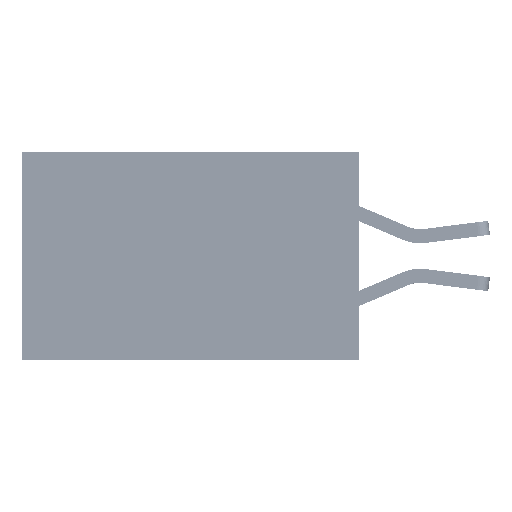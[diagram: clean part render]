
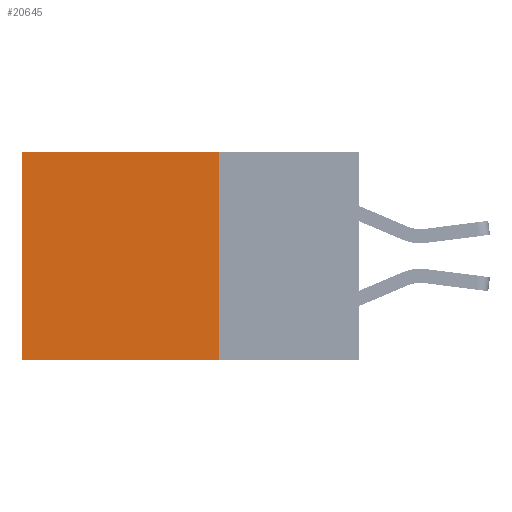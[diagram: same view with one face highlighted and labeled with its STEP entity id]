
A CAD part, left-side view. The second image highlights one B-rep face of the part: STEP entity #20645.
In plain terms, the highlighted planar face has unit normal (-1, 0, 0).
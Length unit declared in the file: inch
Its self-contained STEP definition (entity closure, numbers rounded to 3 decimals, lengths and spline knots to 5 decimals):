
#1061 = ORIENTED_EDGE ( 'NONE', *, *, #5730, .F. ) ;
#2067 = DIRECTION ( 'NONE',  ( 0., 1., 0. ) ) ;
#2556 = CARTESIAN_POINT ( 'NONE',  ( 0.2875, 0.25, 0. ) ) ;
#5730 = EDGE_CURVE ( 'NONE', #26366, #42859, #46177, .T. ) ;
#6614 = ORIENTED_EDGE ( 'NONE', *, *, #29179, .T. ) ;
#8830 = ORIENTED_EDGE ( 'NONE', *, *, #38802, .F. ) ;
#8844 = EDGE_LOOP ( 'NONE', ( #39685, #8830, #1061, #6614 ) ) ;
#10442 = DIRECTION ( 'NONE',  ( 0., 0., -1. ) ) ;
#12081 = AXIS2_PLACEMENT_3D ( 'NONE', #20845, #13208, #27325 ) ;
#13208 = DIRECTION ( 'NONE',  ( 1., 0., 0. ) ) ;
#13329 = CARTESIAN_POINT ( 'NONE',  ( 0.2875, 0.25, 0. ) ) ;
#16786 = PLANE ( 'NONE',  #12081 ) ;
#19938 = LINE ( 'NONE', #27145, #25072 ) ;
#20645 = ADVANCED_FACE ( 'NONE', ( #46052 ), #16786, .F. ) ;
#20845 = CARTESIAN_POINT ( 'NONE',  ( 0.2875, 0.25, 0. ) ) ;
#23786 = CARTESIAN_POINT ( 'NONE',  ( 0.2875, 0.25, -0.37 ) ) ;
#25072 = VECTOR ( 'NONE', #34359, 39.37008 ) ;
#25984 = CARTESIAN_POINT ( 'NONE',  ( 0.2875, 0.6, -0.37 ) ) ;
#26366 = VERTEX_POINT ( 'NONE', #41439 ) ;
#27145 = CARTESIAN_POINT ( 'NONE',  ( 0.2875, 0.25, -0.37 ) ) ;
#27325 = DIRECTION ( 'NONE',  ( 0., 0., -1. ) ) ;
#27928 = DIRECTION ( 'NONE',  ( 0., 0., -1. ) ) ;
#28674 = VERTEX_POINT ( 'NONE', #25984 ) ;
#29179 = EDGE_CURVE ( 'NONE', #26366, #43064, #31343, .T. ) ;
#29531 = CARTESIAN_POINT ( 'NONE',  ( 0.2875, 0.6, 0. ) ) ;
#31065 = VECTOR ( 'NONE', #10442, 39.37008 ) ;
#31343 = LINE ( 'NONE', #2556, #36084 ) ;
#32749 = CARTESIAN_POINT ( 'NONE',  ( 0.2875, 0.6, 0. ) ) ;
#34294 = EDGE_CURVE ( 'NONE', #43064, #28674, #40191, .T. ) ;
#34359 = DIRECTION ( 'NONE',  ( 0., 1., 0. ) ) ;
#36084 = VECTOR ( 'NONE', #2067, 39.37008 ) ;
#38802 = EDGE_CURVE ( 'NONE', #42859, #28674, #19938, .T. ) ;
#39685 = ORIENTED_EDGE ( 'NONE', *, *, #34294, .T. ) ;
#40191 = LINE ( 'NONE', #32749, #31065 ) ;
#41439 = CARTESIAN_POINT ( 'NONE',  ( 0.2875, 0.25, 0. ) ) ;
#42859 = VERTEX_POINT ( 'NONE', #23786 ) ;
#43064 = VERTEX_POINT ( 'NONE', #29531 ) ;
#45304 = VECTOR ( 'NONE', #27928, 39.37008 ) ;
#46052 = FACE_OUTER_BOUND ( 'NONE', #8844, .T. ) ;
#46177 = LINE ( 'NONE', #13329, #45304 ) ;
